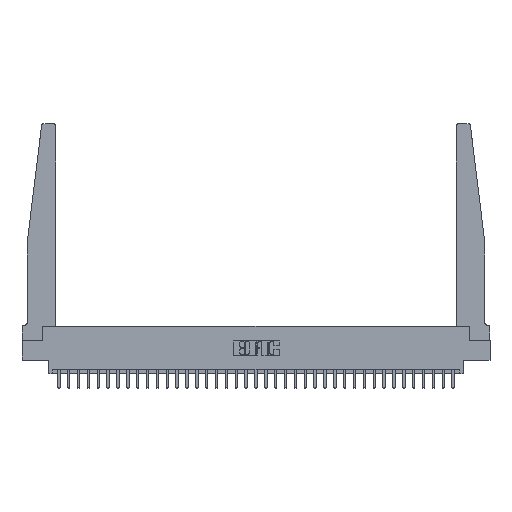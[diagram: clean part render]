
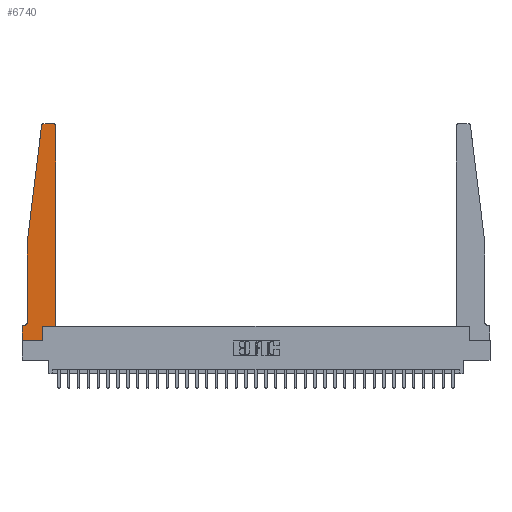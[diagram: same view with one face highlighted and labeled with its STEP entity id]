
A CAD part, top view. The second image highlights one B-rep face of the part: STEP entity #6740.
In plain terms, the highlighted planar face has unit normal (0, 0, 1).
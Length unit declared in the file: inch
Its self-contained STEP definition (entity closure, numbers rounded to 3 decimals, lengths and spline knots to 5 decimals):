
#1028 = DIRECTION ( 'NONE',  ( 0., 1., 0. ) ) ;
#1053 = EDGE_CURVE ( 'NONE', #3104, #5930, #11038, .T. ) ;
#1100 = CIRCLE ( 'NONE', #22738, 0.03 ) ;
#1125 = CARTESIAN_POINT ( 'NONE',  ( 0., 0., 0.37 ) ) ;
#1638 = CARTESIAN_POINT ( 'NONE',  ( 0.065, 1.25, 0.37 ) ) ;
#1747 = CIRCLE ( 'NONE', #23289, 0.03 ) ;
#2043 = CARTESIAN_POINT ( 'NONE',  ( 0.425, 0.18, 0.37 ) ) ;
#2849 = CARTESIAN_POINT ( 'NONE',  ( 0.395, 2.72, 0.37 ) ) ;
#2895 = CARTESIAN_POINT ( 'NONE',  ( 0.395, 2.75, 0.37 ) ) ;
#2912 = VECTOR ( 'NONE', #21551, 39.37008 ) ;
#3030 = LINE ( 'NONE', #11022, #29316 ) ;
#3055 = DIRECTION ( 'NONE',  ( -0.122, -0.992, 0. ) ) ;
#3104 = VERTEX_POINT ( 'NONE', #28324 ) ;
#3362 = VECTOR ( 'NONE', #6155, 39.37008 ) ;
#3372 = CARTESIAN_POINT ( 'NONE',  ( 0.065, 1.25, 0.37 ) ) ;
#3585 = EDGE_CURVE ( 'NONE', #31490, #20046, #3030, .T. ) ;
#4286 = VECTOR ( 'NONE', #3055, 39.37008 ) ;
#4829 = VECTOR ( 'NONE', #6692, 39.37008 ) ;
#5355 = CARTESIAN_POINT ( 'NONE',  ( 0.2605, 0.18, 0.37 ) ) ;
#5383 = DIRECTION ( 'NONE',  ( 1., 0., 0. ) ) ;
#5930 = VERTEX_POINT ( 'NONE', #9759 ) ;
#5936 = EDGE_CURVE ( 'NONE', #9664, #25313, #18616, .T. ) ;
#6155 = DIRECTION ( 'NONE',  ( 0., -1., 0. ) ) ;
#6680 = DIRECTION ( 'NONE',  ( 0., 0., 1. ) ) ;
#6692 = DIRECTION ( 'NONE',  ( 0., -1., 0. ) ) ;
#6740 = ADVANCED_FACE ( 'NONE', ( #19173 ), #28040, .T. ) ;
#6742 = LINE ( 'NONE', #25741, #19295 ) ;
#6852 = CARTESIAN_POINT ( 'NONE',  ( 0.425, 0.18, 0.37 ) ) ;
#7084 = ORIENTED_EDGE ( 'NONE', *, *, #13426, .T. ) ;
#7318 = ORIENTED_EDGE ( 'NONE', *, *, #5936, .T. ) ;
#7466 = EDGE_CURVE ( 'NONE', #20276, #3104, #1100, .T. ) ;
#7698 = DIRECTION ( 'NONE',  ( 0., 0., -1. ) ) ;
#7786 = ORIENTED_EDGE ( 'NONE', *, *, #14716, .T. ) ;
#7834 = ORIENTED_EDGE ( 'NONE', *, *, #28624, .T. ) ;
#7853 = CARTESIAN_POINT ( 'NONE',  ( 0.425, 2.72, 0.37 ) ) ;
#9664 = VERTEX_POINT ( 'NONE', #18098 ) ;
#9759 = CARTESIAN_POINT ( 'NONE',  ( 0.065, 1.25, 0.37 ) ) ;
#10842 = CARTESIAN_POINT ( 'NONE',  ( 0., 0.1875, 0.37 ) ) ;
#11022 = CARTESIAN_POINT ( 'NONE',  ( 0.2605, 0.18, 0.37 ) ) ;
#11038 = LINE ( 'NONE', #3372, #4286 ) ;
#11094 = ORIENTED_EDGE ( 'NONE', *, *, #11676, .T. ) ;
#11383 = ORIENTED_EDGE ( 'NONE', *, *, #1053, .T. ) ;
#11676 = EDGE_CURVE ( 'NONE', #30816, #9664, #31332, .T. ) ;
#12159 = ORIENTED_EDGE ( 'NONE', *, *, #7466, .T. ) ;
#12246 = EDGE_CURVE ( 'NONE', #20046, #21015, #24251, .T. ) ;
#12257 = CARTESIAN_POINT ( 'NONE',  ( 0., 0., 0.37 ) ) ;
#13426 = EDGE_CURVE ( 'NONE', #27398, #20276, #24543, .T. ) ;
#13476 = DIRECTION ( 'NONE',  ( 1., 0., 0. ) ) ;
#13765 = EDGE_LOOP ( 'NONE', ( #7084, #12159, #11383, #7834, #11094, #7318, #7786, #29772, #27155, #26348, #25970, #24836 ) ) ;
#13952 = VERTEX_POINT ( 'NONE', #7853 ) ;
#14716 = EDGE_CURVE ( 'NONE', #25313, #22729, #16733, .T. ) ;
#15899 = CARTESIAN_POINT ( 'NONE',  ( 0.25, 2.75, 0.37 ) ) ;
#15964 = DIRECTION ( 'NONE',  ( 0., 1., 0. ) ) ;
#16223 = CARTESIAN_POINT ( 'NONE',  ( 0.27653, 2.75, 0.37 ) ) ;
#16733 = LINE ( 'NONE', #1125, #3362 ) ;
#17341 = CARTESIAN_POINT ( 'NONE',  ( 0.065, 0.1875, 0.37 ) ) ;
#18098 = CARTESIAN_POINT ( 'NONE',  ( 0.015, 0.1875, 0.37 ) ) ;
#18616 = LINE ( 'NONE', #17341, #23609 ) ;
#19004 = LINE ( 'NONE', #1638, #4829 ) ;
#19045 = CARTESIAN_POINT ( 'NONE',  ( 0., 0., 0.37 ) ) ;
#19173 = FACE_OUTER_BOUND ( 'NONE', #13765, .T. ) ;
#19295 = VECTOR ( 'NONE', #15964, 39.37008 ) ;
#20039 = CARTESIAN_POINT ( 'NONE',  ( 0., 0.1875, 0.37 ) ) ;
#20046 = VERTEX_POINT ( 'NONE', #5355 ) ;
#20276 = VERTEX_POINT ( 'NONE', #16223 ) ;
#20323 = AXIS2_PLACEMENT_3D ( 'NONE', #22674, #7698, #25067 ) ;
#20412 = DIRECTION ( 'NONE',  ( 0., 0., 1. ) ) ;
#21015 = VERTEX_POINT ( 'NONE', #6852 ) ;
#21551 = DIRECTION ( 'NONE',  ( 1., 0., 0. ) ) ;
#21689 = CARTESIAN_POINT ( 'NONE',  ( 0.27653, 2.72, 0.37 ) ) ;
#22674 = CARTESIAN_POINT ( 'NONE',  ( 0.015, 0.2375, 0.37 ) ) ;
#22729 = VERTEX_POINT ( 'NONE', #12257 ) ;
#22738 = AXIS2_PLACEMENT_3D ( 'NONE', #21689, #6680, #24109 ) ;
#22895 = LINE ( 'NONE', #19045, #2912 ) ;
#23289 = AXIS2_PLACEMENT_3D ( 'NONE', #2849, #20412, #5383 ) ;
#23512 = VECTOR ( 'NONE', #24402, 39.37008 ) ;
#23609 = VECTOR ( 'NONE', #29403, 39.37008 ) ;
#23813 = VECTOR ( 'NONE', #25692, 39.37008 ) ;
#24109 = DIRECTION ( 'NONE',  ( 1., 0., 0. ) ) ;
#24251 = LINE ( 'NONE', #2043, #23512 ) ;
#24402 = DIRECTION ( 'NONE',  ( 1., 0., 0. ) ) ;
#24430 = EDGE_CURVE ( 'NONE', #22729, #31490, #22895, .T. ) ;
#24543 = LINE ( 'NONE', #15899, #23813 ) ;
#24836 = ORIENTED_EDGE ( 'NONE', *, *, #28313, .T. ) ;
#25067 = DIRECTION ( 'NONE',  ( -1., 0., 0. ) ) ;
#25313 = VERTEX_POINT ( 'NONE', #20039 ) ;
#25544 = AXIS2_PLACEMENT_3D ( 'NONE', #10842, #28140, #13476 ) ;
#25692 = DIRECTION ( 'NONE',  ( -1., 0., 0. ) ) ;
#25741 = CARTESIAN_POINT ( 'NONE',  ( 0.425, 0.18, 0.37 ) ) ;
#25970 = ORIENTED_EDGE ( 'NONE', *, *, #26179, .T. ) ;
#26179 = EDGE_CURVE ( 'NONE', #21015, #13952, #6742, .T. ) ;
#26348 = ORIENTED_EDGE ( 'NONE', *, *, #12246, .T. ) ;
#27155 = ORIENTED_EDGE ( 'NONE', *, *, #3585, .T. ) ;
#27398 = VERTEX_POINT ( 'NONE', #2895 ) ;
#27556 = CARTESIAN_POINT ( 'NONE',  ( 0.065, 0.2375, 0.37 ) ) ;
#28040 = PLANE ( 'NONE',  #25544 ) ;
#28140 = DIRECTION ( 'NONE',  ( 0., 0., 1. ) ) ;
#28313 = EDGE_CURVE ( 'NONE', #13952, #27398, #1747, .T. ) ;
#28324 = CARTESIAN_POINT ( 'NONE',  ( 0.24675, 2.72367, 0.37 ) ) ;
#28624 = EDGE_CURVE ( 'NONE', #5930, #30816, #19004, .T. ) ;
#29316 = VECTOR ( 'NONE', #1028, 39.37008 ) ;
#29403 = DIRECTION ( 'NONE',  ( -1., 0., 0. ) ) ;
#29772 = ORIENTED_EDGE ( 'NONE', *, *, #24430, .T. ) ;
#30816 = VERTEX_POINT ( 'NONE', #27556 ) ;
#31136 = CARTESIAN_POINT ( 'NONE',  ( 0.2605, 0., 0.37 ) ) ;
#31332 = CIRCLE ( 'NONE', #20323, 0.05 ) ;
#31490 = VERTEX_POINT ( 'NONE', #31136 ) ;
